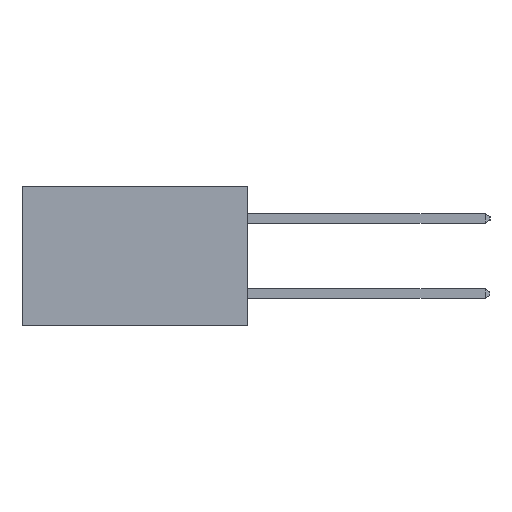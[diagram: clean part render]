
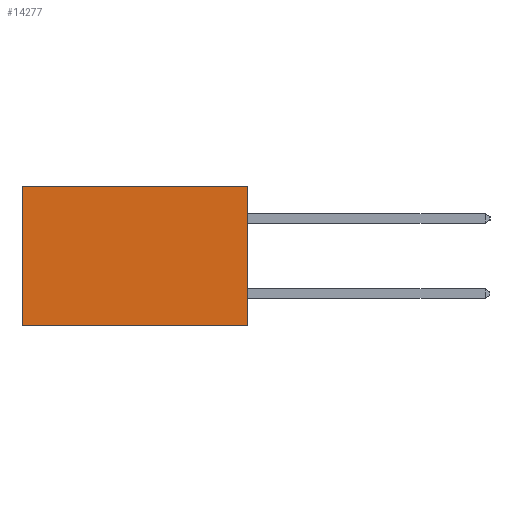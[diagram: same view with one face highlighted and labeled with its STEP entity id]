
A CAD part, left-side view. The second image highlights one B-rep face of the part: STEP entity #14277.
In plain terms, the highlighted planar face has unit normal (-1, 0, 0).
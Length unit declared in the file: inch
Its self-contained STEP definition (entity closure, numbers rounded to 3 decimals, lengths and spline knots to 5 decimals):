
#56 = DIRECTION ( 'NONE',  ( 0., 0., -1. ) ) ;
#68 = ORIENTED_EDGE ( 'NONE', *, *, #3265, .T. ) ;
#943 = ORIENTED_EDGE ( 'NONE', *, *, #9762, .T. ) ;
#1119 = EDGE_LOOP ( 'NONE', ( #68, #2046, #9556, #943 ) ) ;
#1983 = VERTEX_POINT ( 'NONE', #4648 ) ;
#2046 = ORIENTED_EDGE ( 'NONE', *, *, #16123, .F. ) ;
#2568 = VECTOR ( 'NONE', #56, 39.37008 ) ;
#3265 = EDGE_CURVE ( 'NONE', #8978, #11325, #13136, .T. ) ;
#3296 = CARTESIAN_POINT ( 'NONE',  ( 0.298, 0.6, -0.37 ) ) ;
#3911 = CARTESIAN_POINT ( 'NONE',  ( 0.298, 0.6, 0. ) ) ;
#4648 = CARTESIAN_POINT ( 'NONE',  ( 0.298, 0., 0. ) ) ;
#5471 = CARTESIAN_POINT ( 'NONE',  ( 0.298, 0., -0.37 ) ) ;
#5577 = DIRECTION ( 'NONE',  ( 0., 0., -1. ) ) ;
#5998 = DIRECTION ( 'NONE',  ( 0., 1., 0. ) ) ;
#6739 = LINE ( 'NONE', #14861, #16542 ) ;
#6854 = CARTESIAN_POINT ( 'NONE',  ( 0.298, 0., 0. ) ) ;
#7876 = VECTOR ( 'NONE', #5998, 39.37008 ) ;
#8528 = CARTESIAN_POINT ( 'NONE',  ( 0.298, 0.6, 0. ) ) ;
#8608 = CARTESIAN_POINT ( 'NONE',  ( 0.298, 0., -0.37 ) ) ;
#8718 = DIRECTION ( 'NONE',  ( 0., 0., -1. ) ) ;
#8978 = VERTEX_POINT ( 'NONE', #3911 ) ;
#9556 = ORIENTED_EDGE ( 'NONE', *, *, #13072, .F. ) ;
#9762 = EDGE_CURVE ( 'NONE', #1983, #8978, #6739, .T. ) ;
#10925 = VECTOR ( 'NONE', #5577, 39.37008 ) ;
#11325 = VERTEX_POINT ( 'NONE', #3296 ) ;
#11913 = AXIS2_PLACEMENT_3D ( 'NONE', #12583, #16337, #8718 ) ;
#12400 = VERTEX_POINT ( 'NONE', #5471 ) ;
#12583 = CARTESIAN_POINT ( 'NONE',  ( 0.298, 0., 0. ) ) ;
#13072 = EDGE_CURVE ( 'NONE', #1983, #12400, #14758, .T. ) ;
#13136 = LINE ( 'NONE', #8528, #2568 ) ;
#13209 = FACE_OUTER_BOUND ( 'NONE', #1119, .T. ) ;
#14277 = ADVANCED_FACE ( 'NONE', ( #13209 ), #15153, .F. ) ;
#14758 = LINE ( 'NONE', #6854, #10925 ) ;
#14842 = DIRECTION ( 'NONE',  ( 0., 1., 0. ) ) ;
#14861 = CARTESIAN_POINT ( 'NONE',  ( 0.298, 0., 0. ) ) ;
#15153 = PLANE ( 'NONE',  #11913 ) ;
#15154 = LINE ( 'NONE', #8608, #7876 ) ;
#16123 = EDGE_CURVE ( 'NONE', #12400, #11325, #15154, .T. ) ;
#16337 = DIRECTION ( 'NONE',  ( 1., 0., 0. ) ) ;
#16542 = VECTOR ( 'NONE', #14842, 39.37008 ) ;
